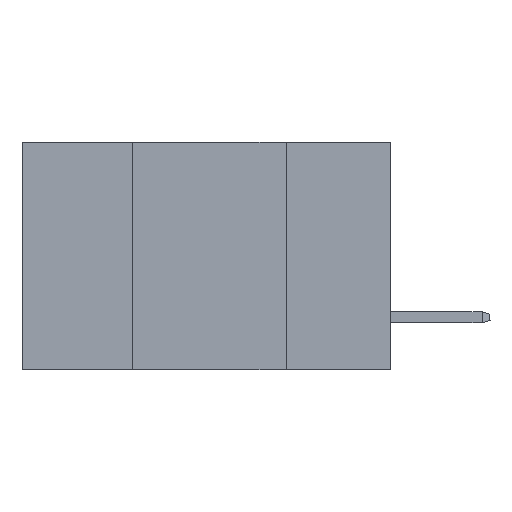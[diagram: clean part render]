
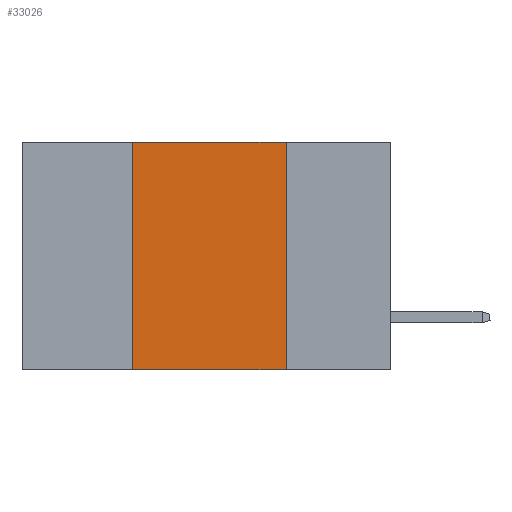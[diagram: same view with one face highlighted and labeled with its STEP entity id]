
A CAD part, left-side view. The second image highlights one B-rep face of the part: STEP entity #33026.
In plain terms, the highlighted planar face has unit normal (-1, 0, 0).
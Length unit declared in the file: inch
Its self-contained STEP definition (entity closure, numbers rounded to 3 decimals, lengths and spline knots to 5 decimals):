
#812 = AXIS2_PLACEMENT_3D ( 'NONE', #18051, #13025, #10303 ) ;
#887 = CARTESIAN_POINT ( 'NONE',  ( 0., 0.42, -0.37 ) ) ;
#1950 = PLANE ( 'NONE',  #812 ) ;
#2268 = LINE ( 'NONE', #25719, #27499 ) ;
#3387 = VECTOR ( 'NONE', #28835, 39.37008 ) ;
#3860 = FACE_OUTER_BOUND ( 'NONE', #26004, .T. ) ;
#6942 = CARTESIAN_POINT ( 'NONE',  ( 0., 0.17, 0. ) ) ;
#9037 = DIRECTION ( 'NONE',  ( 0., -1., 0. ) ) ;
#9376 = EDGE_CURVE ( 'NONE', #22307, #24868, #15775, .T. ) ;
#9725 = ORIENTED_EDGE ( 'NONE', *, *, #15979, .F. ) ;
#9866 = VECTOR ( 'NONE', #21195, 39.37008 ) ;
#10303 = DIRECTION ( 'NONE',  ( 0., 0., -1. ) ) ;
#10673 = LINE ( 'NONE', #22450, #16138 ) ;
#10828 = ORIENTED_EDGE ( 'NONE', *, *, #11035, .F. ) ;
#11035 = EDGE_CURVE ( 'NONE', #30045, #17172, #13122, .T. ) ;
#12324 = DIRECTION ( 'NONE',  ( 0., -1., 0. ) ) ;
#13025 = DIRECTION ( 'NONE',  ( 1., 0., 0. ) ) ;
#13122 = LINE ( 'NONE', #6942, #3387 ) ;
#15775 = LINE ( 'NONE', #24467, #9866 ) ;
#15979 = EDGE_CURVE ( 'NONE', #24868, #30045, #10673, .T. ) ;
#16138 = VECTOR ( 'NONE', #9037, 39.37008 ) ;
#17172 = VERTEX_POINT ( 'NONE', #30666 ) ;
#18051 = CARTESIAN_POINT ( 'NONE',  ( 0., 0.6, 0. ) ) ;
#21106 = EDGE_CURVE ( 'NONE', #22307, #17172, #2268, .T. ) ;
#21195 = DIRECTION ( 'NONE',  ( 0., 0., 1. ) ) ;
#22307 = VERTEX_POINT ( 'NONE', #887 ) ;
#22450 = CARTESIAN_POINT ( 'NONE',  ( 0., 0.6, 0. ) ) ;
#24467 = CARTESIAN_POINT ( 'NONE',  ( 0., 0.42, 0. ) ) ;
#24868 = VERTEX_POINT ( 'NONE', #30730 ) ;
#25719 = CARTESIAN_POINT ( 'NONE',  ( 0., 0.6, -0.37 ) ) ;
#26004 = EDGE_LOOP ( 'NONE', ( #10828, #9725, #28886, #31870 ) ) ;
#26325 = CARTESIAN_POINT ( 'NONE',  ( 0., 0.17, 0. ) ) ;
#27499 = VECTOR ( 'NONE', #12324, 39.37008 ) ;
#28835 = DIRECTION ( 'NONE',  ( 0., 0., -1. ) ) ;
#28886 = ORIENTED_EDGE ( 'NONE', *, *, #9376, .F. ) ;
#30045 = VERTEX_POINT ( 'NONE', #26325 ) ;
#30666 = CARTESIAN_POINT ( 'NONE',  ( 0., 0.17, -0.37 ) ) ;
#30730 = CARTESIAN_POINT ( 'NONE',  ( 0., 0.42, 0. ) ) ;
#31870 = ORIENTED_EDGE ( 'NONE', *, *, #21106, .T. ) ;
#33026 = ADVANCED_FACE ( 'NONE', ( #3860 ), #1950, .F. ) ;
